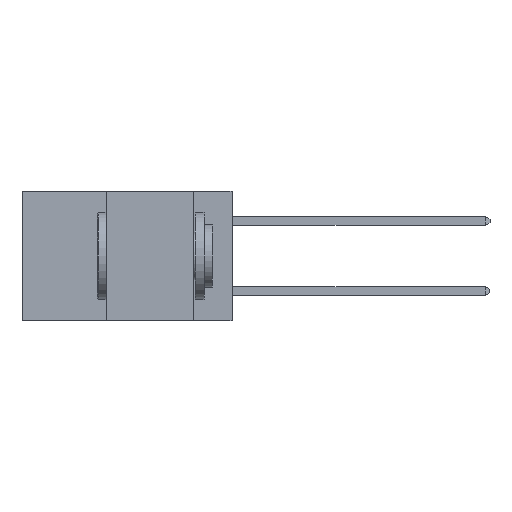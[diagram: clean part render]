
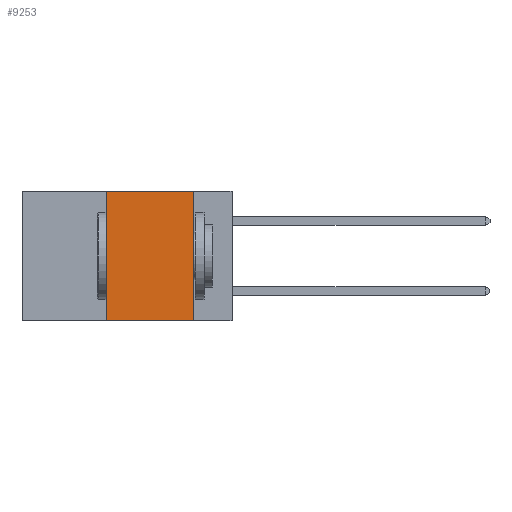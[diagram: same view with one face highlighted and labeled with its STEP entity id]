
A CAD part, left-side view. The second image highlights one B-rep face of the part: STEP entity #9253.
In plain terms, the highlighted planar face has unit normal (-1, 0, 0).
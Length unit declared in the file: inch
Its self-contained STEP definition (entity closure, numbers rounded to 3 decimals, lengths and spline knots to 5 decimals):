
#288 = ORIENTED_EDGE ( 'NONE', *, *, #12850, .F. ) ;
#319 = ORIENTED_EDGE ( 'NONE', *, *, #13876, .F. ) ;
#337 = EDGE_CURVE ( 'NONE', #6381, #16239, #12603, .T. ) ;
#487 = ORIENTED_EDGE ( 'NONE', *, *, #16162, .F. ) ;
#491 = ORIENTED_EDGE ( 'NONE', *, *, #337, .T. ) ;
#725 = VECTOR ( 'NONE', #14363, 39.37008 ) ;
#1791 = CARTESIAN_POINT ( 'NONE',  ( 0., 0.11, 0. ) ) ;
#2430 = VECTOR ( 'NONE', #7406, 39.37008 ) ;
#3314 = EDGE_LOOP ( 'NONE', ( #288, #319, #487, #491 ) ) ;
#3674 = VECTOR ( 'NONE', #4366, 39.37008 ) ;
#3981 = FACE_OUTER_BOUND ( 'NONE', #3314, .T. ) ;
#4366 = DIRECTION ( 'NONE',  ( 0., 0., -1. ) ) ;
#5235 = VERTEX_POINT ( 'NONE', #14710 ) ;
#5847 = VECTOR ( 'NONE', #11651, 39.37008 ) ;
#6325 = DIRECTION ( 'NONE',  ( 0., 0., -1. ) ) ;
#6381 = VERTEX_POINT ( 'NONE', #15963 ) ;
#7008 = LINE ( 'NONE', #1791, #3674 ) ;
#7406 = DIRECTION ( 'NONE',  ( 0., -1., 0. ) ) ;
#9111 = LINE ( 'NONE', #11197, #2430 ) ;
#9253 = ADVANCED_FACE ( 'NONE', ( #3981 ), #12709, .F. ) ;
#9881 = CARTESIAN_POINT ( 'NONE',  ( 0., 0.36, 0. ) ) ;
#10402 = CARTESIAN_POINT ( 'NONE',  ( 0., 0.36, 0. ) ) ;
#11197 = CARTESIAN_POINT ( 'NONE',  ( 0., 0.6, 0. ) ) ;
#11535 = CARTESIAN_POINT ( 'NONE',  ( 0., 0.6, -0.37 ) ) ;
#11651 = DIRECTION ( 'NONE',  ( 0., -1., 0. ) ) ;
#12603 = LINE ( 'NONE', #11535, #5847 ) ;
#12709 = PLANE ( 'NONE',  #15092 ) ;
#12850 = EDGE_CURVE ( 'NONE', #5235, #16239, #7008, .T. ) ;
#13876 = EDGE_CURVE ( 'NONE', #13924, #5235, #9111, .T. ) ;
#13924 = VERTEX_POINT ( 'NONE', #9881 ) ;
#14039 = DIRECTION ( 'NONE',  ( 1., 0., 0. ) ) ;
#14344 = LINE ( 'NONE', #10402, #725 ) ;
#14363 = DIRECTION ( 'NONE',  ( 0., 0., 1. ) ) ;
#14536 = CARTESIAN_POINT ( 'NONE',  ( 0., 0.11, -0.37 ) ) ;
#14710 = CARTESIAN_POINT ( 'NONE',  ( 0., 0.11, 0. ) ) ;
#15092 = AXIS2_PLACEMENT_3D ( 'NONE', #16602, #14039, #6325 ) ;
#15963 = CARTESIAN_POINT ( 'NONE',  ( 0., 0.36, -0.37 ) ) ;
#16162 = EDGE_CURVE ( 'NONE', #6381, #13924, #14344, .T. ) ;
#16239 = VERTEX_POINT ( 'NONE', #14536 ) ;
#16602 = CARTESIAN_POINT ( 'NONE',  ( 0., 0.6, 0. ) ) ;
